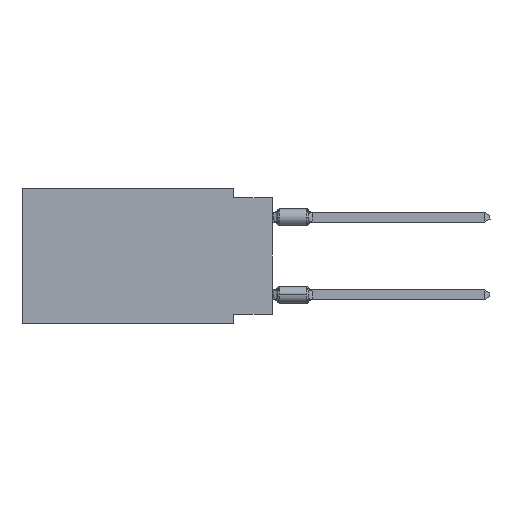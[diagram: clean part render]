
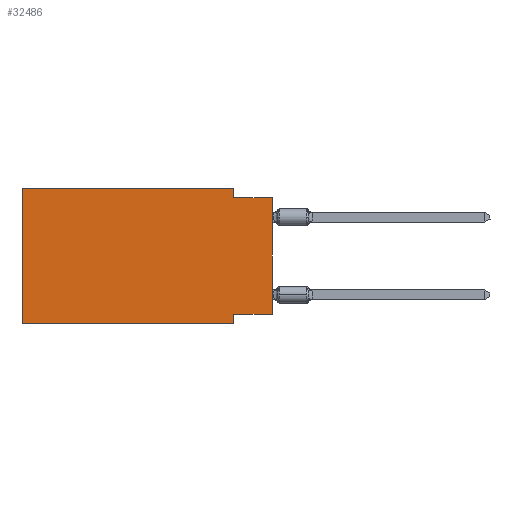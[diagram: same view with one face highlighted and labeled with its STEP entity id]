
A CAD part, left-side view. The second image highlights one B-rep face of the part: STEP entity #32486.
In plain terms, the highlighted planar face has unit normal (-1, 0, 0).
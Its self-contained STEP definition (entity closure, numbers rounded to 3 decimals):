
#400 = CARTESIAN_POINT ( 'NONE',  ( 0., 2.54, 0. ) ) ;
#886 = CARTESIAN_POINT ( 'NONE',  ( 0., 2.54, -8.255 ) ) ;
#3582 = VERTEX_POINT ( 'NONE', #46659 ) ;
#3971 = VERTEX_POINT ( 'NONE', #886 ) ;
#4503 = DIRECTION ( 'NONE',  ( 0., -1., 0. ) ) ;
#4804 = VERTEX_POINT ( 'NONE', #47813 ) ;
#5089 = DIRECTION ( 'NONE',  ( 0., 0., 1. ) ) ;
#5641 = CARTESIAN_POINT ( 'NONE',  ( 0., 2.54, -8.89 ) ) ;
#5663 = CARTESIAN_POINT ( 'NONE',  ( 0., 2.54, -8.89 ) ) ;
#5691 = LINE ( 'NONE', #28754, #13734 ) ;
#6431 = DIRECTION ( 'NONE',  ( 1., 0., 0. ) ) ;
#6789 = DIRECTION ( 'NONE',  ( 0., 1., 0. ) ) ;
#7021 = VECTOR ( 'NONE', #4503, 1000. ) ;
#7503 = VECTOR ( 'NONE', #5089, 1000. ) ;
#8052 = VECTOR ( 'NONE', #37121, 1000. ) ;
#8352 = LINE ( 'NONE', #39586, #7021 ) ;
#10532 = FACE_OUTER_BOUND ( 'NONE', #22307, .T. ) ;
#10886 = CARTESIAN_POINT ( 'NONE',  ( 0., 0., -8.255 ) ) ;
#11635 = CARTESIAN_POINT ( 'NONE',  ( 0., 0., -8.255 ) ) ;
#12264 = EDGE_CURVE ( 'NONE', #3582, #17271, #45993, .T. ) ;
#13734 = VECTOR ( 'NONE', #21562, 1000. ) ;
#14056 = EDGE_CURVE ( 'NONE', #19545, #3971, #14976, .T. ) ;
#14976 = LINE ( 'NONE', #10886, #18098 ) ;
#15205 = VERTEX_POINT ( 'NONE', #30875 ) ;
#16444 = LINE ( 'NONE', #23873, #32673 ) ;
#17271 = VERTEX_POINT ( 'NONE', #5641 ) ;
#18040 = EDGE_CURVE ( 'NONE', #50125, #41081, #8352, .T. ) ;
#18098 = VECTOR ( 'NONE', #6789, 1000. ) ;
#19545 = VERTEX_POINT ( 'NONE', #11635 ) ;
#20362 = EDGE_CURVE ( 'NONE', #4804, #15205, #5691, .T. ) ;
#20804 = EDGE_CURVE ( 'NONE', #41081, #4804, #44292, .T. ) ;
#21562 = DIRECTION ( 'NONE',  ( 0., -1., 0. ) ) ;
#22307 = EDGE_LOOP ( 'NONE', ( #25228, #23259, #28243, #23866, #23246, #44644, #29810, #37861 ) ) ;
#23212 = CARTESIAN_POINT ( 'NONE',  ( 0., 16.383, -8.89 ) ) ;
#23246 = ORIENTED_EDGE ( 'NONE', *, *, #44469, .F. ) ;
#23259 = ORIENTED_EDGE ( 'NONE', *, *, #20362, .F. ) ;
#23866 = ORIENTED_EDGE ( 'NONE', *, *, #18040, .F. ) ;
#23873 = CARTESIAN_POINT ( 'NONE',  ( 0., 0., 0. ) ) ;
#25150 = LINE ( 'NONE', #5663, #49391 ) ;
#25228 = ORIENTED_EDGE ( 'NONE', *, *, #48172, .T. ) ;
#26109 = AXIS2_PLACEMENT_3D ( 'NONE', #33823, #6431, #37909 ) ;
#28243 = ORIENTED_EDGE ( 'NONE', *, *, #20804, .F. ) ;
#28440 = CARTESIAN_POINT ( 'NONE',  ( 0., 2.54, 0. ) ) ;
#28754 = CARTESIAN_POINT ( 'NONE',  ( 0., 0., -0.635 ) ) ;
#29179 = LINE ( 'NONE', #40173, #7503 ) ;
#29497 = PLANE ( 'NONE',  #26109 ) ;
#29810 = ORIENTED_EDGE ( 'NONE', *, *, #31362, .F. ) ;
#30875 = CARTESIAN_POINT ( 'NONE',  ( 0., 0., -0.635 ) ) ;
#31362 = EDGE_CURVE ( 'NONE', #3971, #17271, #25150, .T. ) ;
#32486 = ADVANCED_FACE ( 'NONE', ( #10532 ), #29497, .F. ) ;
#32673 = VECTOR ( 'NONE', #36152, 1000. ) ;
#33823 = CARTESIAN_POINT ( 'NONE',  ( 0., 16.383, 0. ) ) ;
#34967 = CARTESIAN_POINT ( 'NONE',  ( 0., 16.383, 0. ) ) ;
#36152 = DIRECTION ( 'NONE',  ( 0., 0., 1. ) ) ;
#37121 = DIRECTION ( 'NONE',  ( 0., 0., -1. ) ) ;
#37414 = DIRECTION ( 'NONE',  ( 0., 0., -1. ) ) ;
#37861 = ORIENTED_EDGE ( 'NONE', *, *, #14056, .F. ) ;
#37909 = DIRECTION ( 'NONE',  ( 0., 0., -1. ) ) ;
#39586 = CARTESIAN_POINT ( 'NONE',  ( 0., 16.383, 0. ) ) ;
#40173 = CARTESIAN_POINT ( 'NONE',  ( 0., 16.383, 0. ) ) ;
#41081 = VERTEX_POINT ( 'NONE', #400 ) ;
#44292 = LINE ( 'NONE', #28440, #8052 ) ;
#44469 = EDGE_CURVE ( 'NONE', #3582, #50125, #29179, .T. ) ;
#44644 = ORIENTED_EDGE ( 'NONE', *, *, #12264, .T. ) ;
#45993 = LINE ( 'NONE', #23212, #46736 ) ;
#46659 = CARTESIAN_POINT ( 'NONE',  ( 0., 16.383, -8.89 ) ) ;
#46736 = VECTOR ( 'NONE', #49592, 1000. ) ;
#47813 = CARTESIAN_POINT ( 'NONE',  ( 0., 2.54, -0.635 ) ) ;
#48172 = EDGE_CURVE ( 'NONE', #19545, #15205, #16444, .T. ) ;
#49391 = VECTOR ( 'NONE', #37414, 1000. ) ;
#49592 = DIRECTION ( 'NONE',  ( 0., -1., 0. ) ) ;
#50125 = VERTEX_POINT ( 'NONE', #34967 ) ;
